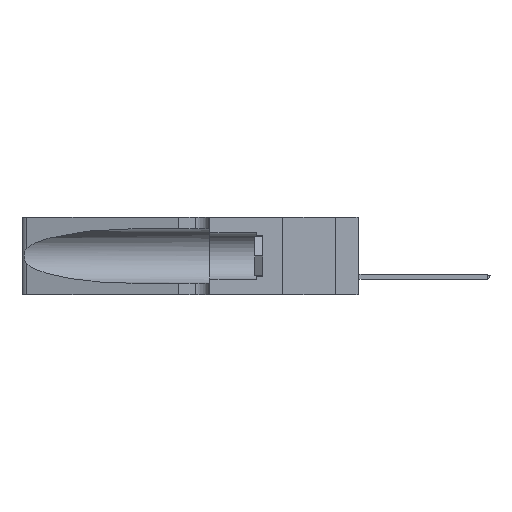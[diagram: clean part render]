
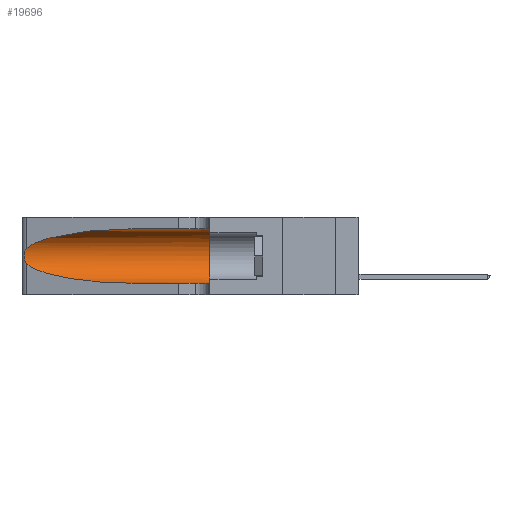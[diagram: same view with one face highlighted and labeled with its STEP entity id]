
A CAD part, left-side view. The second image highlights one B-rep face of the part: STEP entity #19696.
In plain terms, the highlighted cylindrical face has radius 3.308 mm (diameter 6.617 mm), a partial arc.
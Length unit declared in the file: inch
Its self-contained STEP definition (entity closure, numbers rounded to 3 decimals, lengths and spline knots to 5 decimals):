
#3224 = EDGE_CURVE ( 'NONE', #7602, #28068, #20324, .T. ) ;
#3632 = VERTEX_POINT ( 'NONE', #48541 ) ;
#4556 = EDGE_CURVE ( 'NONE', #50228, #3632, #8277, .T. ) ;
#5064 = DIRECTION ( 'NONE',  ( 0., 0., -1. ) ) ;
#5719 = FACE_OUTER_BOUND ( 'NONE', #31353, .T. ) ;
#6434 = CARTESIAN_POINT ( 'NONE',  ( 0.25639, 1.23184, 0.21858 ) ) ;
#6555 = AXIS2_PLACEMENT_3D ( 'NONE', #33342, #36722, #5064 ) ;
#7181 = DIRECTION ( 'NONE',  ( 0., -1., 0. ) ) ;
#7602 = VERTEX_POINT ( 'NONE', #30326 ) ;
#8277 = CIRCLE ( 'NONE', #33257, 0.13025 ) ;
#11417 = CARTESIAN_POINT ( 'NONE',  ( 0.18966, 0.96281, 0.05475 ) ) ;
#11422 = VECTOR ( 'NONE', #7181, 39.37008 ) ;
#12770 = VECTOR ( 'NONE', #43205, 39.37008 ) ;
#13550 = CARTESIAN_POINT ( 'NONE',  ( 0.2373, 1.15595, 0.28018 ) ) ;
#14125 = CARTESIAN_POINT ( 'NONE',  ( 0.25487, 1.22718, 0.22369 ) ) ;
#15288 = CARTESIAN_POINT ( 'NONE',  ( 0.1305, 1.61858, 0.31525 ) ) ;
#15460 = CARTESIAN_POINT ( 'NONE',  ( 0.25487, 1.22718, 0.14631 ) ) ;
#16062 = VERTEX_POINT ( 'NONE', #21186 ) ;
#16870 = CARTESIAN_POINT ( 'NONE',  ( 0.25639, 1.23186, 0.15144 ) ) ;
#19055 = CARTESIAN_POINT ( 'NONE',  ( 0.25854, 1.2359, 0.20912 ) ) ;
#19230 = CARTESIAN_POINT ( 'NONE',  ( 0.26075, 1.23896, 0.178 ) ) ;
#19696 = ADVANCED_FACE ( 'NONE', ( #5719 ), #38293, .F. ) ;
#19791 = ORIENTED_EDGE ( 'NONE', *, *, #4556, .F. ) ;
#20324 =( BOUNDED_CURVE ( )  B_SPLINE_CURVE ( 3, ( #29430, #41695, #13550, #21571 ),
 .UNSPECIFIED., .F., .F. ) 
 B_SPLINE_CURVE_WITH_KNOTS ( ( 4, 4 ),
 ( 1.5708, 2.84003 ),
 .UNSPECIFIED. ) 
 CURVE ( )  GEOMETRIC_REPRESENTATION_ITEM ( )  RATIONAL_B_SPLINE_CURVE ( ( 1., 0.87, 0.87, 1. ) ) 
 REPRESENTATION_ITEM ( '' )  );
#20940 =( BOUNDED_CURVE ( )  B_SPLINE_CURVE ( 3, ( #15460, #39589, #11417, #39419 ),
 .UNSPECIFIED., .F., .F. ) 
 B_SPLINE_CURVE_WITH_KNOTS ( ( 4, 4 ),
 ( 3.44316, 4.71239 ),
 .UNSPECIFIED. ) 
 CURVE ( )  GEOMETRIC_REPRESENTATION_ITEM ( )  RATIONAL_B_SPLINE_CURVE ( ( 1., 0.87, 0.87, 1. ) ) 
 REPRESENTATION_ITEM ( '' )  );
#21186 = CARTESIAN_POINT ( 'NONE',  ( 0.1305, 0.72297, 0.05475 ) ) ;
#21363 = EDGE_CURVE ( 'NONE', #28068, #22759, #41120, .T. ) ;
#21571 = CARTESIAN_POINT ( 'NONE',  ( 0.25487, 1.22718, 0.22369 ) ) ;
#22495 = ORIENTED_EDGE ( 'NONE', *, *, #44937, .T. ) ;
#22759 = VERTEX_POINT ( 'NONE', #25134 ) ;
#23254 = CARTESIAN_POINT ( 'NONE',  ( 0.25856, 1.23593, 0.16098 ) ) ;
#25134 = CARTESIAN_POINT ( 'NONE',  ( 0.25487, 1.22718, 0.14631 ) ) ;
#26694 = CARTESIAN_POINT ( 'NONE',  ( 0.26075, 1.23896, 0.19203 ) ) ;
#27233 = LINE ( 'NONE', #15288, #12770 ) ;
#28068 = VERTEX_POINT ( 'NONE', #39539 ) ;
#29221 = ORIENTED_EDGE ( 'NONE', *, *, #3224, .T. ) ;
#29430 = CARTESIAN_POINT ( 'NONE',  ( 0.1305, 0.72297, 0.31525 ) ) ;
#30326 = CARTESIAN_POINT ( 'NONE',  ( 0.1305, 0.72297, 0.31525 ) ) ;
#31324 = CARTESIAN_POINT ( 'NONE',  ( 0.1305, 0.35, 0.185 ) ) ;
#31353 = EDGE_LOOP ( 'NONE', ( #29221, #44229, #22495, #33733, #19791, #46419 ) ) ;
#31357 = CARTESIAN_POINT ( 'NONE',  ( 0.1305, 1.61858, 0.05475 ) ) ;
#33257 = AXIS2_PLACEMENT_3D ( 'NONE', #31324, #39546, #50849 ) ;
#33342 = CARTESIAN_POINT ( 'NONE',  ( 0.1305, 1.61858, 0.185 ) ) ;
#33733 = ORIENTED_EDGE ( 'NONE', *, *, #48502, .T. ) ;
#34178 = CARTESIAN_POINT ( 'NONE',  ( 0.25555, 1.22993, 0.14849 ) ) ;
#36722 = DIRECTION ( 'NONE',  ( 0., -1., 0. ) ) ;
#37525 = CARTESIAN_POINT ( 'NONE',  ( 0.25787, 1.23484, 0.2124 ) ) ;
#38264 = CARTESIAN_POINT ( 'NONE',  ( 0.25555, 1.22994, 0.2215 ) ) ;
#38293 = CYLINDRICAL_SURFACE ( 'NONE', #6555, 0.13025 ) ;
#38805 = CARTESIAN_POINT ( 'NONE',  ( 0.26018, 1.23835, 0.19895 ) ) ;
#39419 = CARTESIAN_POINT ( 'NONE',  ( 0.1305, 0.72297, 0.05475 ) ) ;
#39489 = CARTESIAN_POINT ( 'NONE',  ( 0.25487, 1.22718, 0.14631 ) ) ;
#39539 = CARTESIAN_POINT ( 'NONE',  ( 0.25487, 1.22718, 0.22369 ) ) ;
#39546 = DIRECTION ( 'NONE',  ( 0., 1., 0. ) ) ;
#39589 = CARTESIAN_POINT ( 'NONE',  ( 0.2373, 1.15595, 0.08982 ) ) ;
#41120 = B_SPLINE_CURVE_WITH_KNOTS ( 'NONE', 3,
 ( #14125, #38264, #6434, #37525, #19055, #38805, #26694, #19230, #47148, #23254, #51180, #16870, #34178, #39489 ),
 .UNSPECIFIED., .F., .F.,
 ( 4, 2, 2, 2, 2, 2, 4 ),
 ( 0., 0.00027, 0.00053, 0.00107, 0.0016, 0.00187, 0.00214 ),
 .UNSPECIFIED. ) ;
#41695 = CARTESIAN_POINT ( 'NONE',  ( 0.18966, 0.96281, 0.31525 ) ) ;
#43205 = DIRECTION ( 'NONE',  ( 0., -1., 0. ) ) ;
#44229 = ORIENTED_EDGE ( 'NONE', *, *, #21363, .T. ) ;
#44937 = EDGE_CURVE ( 'NONE', #22759, #16062, #20940, .T. ) ;
#45005 = EDGE_CURVE ( 'NONE', #7602, #50228, #27233, .T. ) ;
#46419 = ORIENTED_EDGE ( 'NONE', *, *, #45005, .F. ) ;
#47148 = CARTESIAN_POINT ( 'NONE',  ( 0.26017, 1.23833, 0.17102 ) ) ;
#48502 = EDGE_CURVE ( 'NONE', #16062, #3632, #48819, .T. ) ;
#48541 = CARTESIAN_POINT ( 'NONE',  ( 0.1305, 0.35, 0.05475 ) ) ;
#48819 = LINE ( 'NONE', #31357, #11422 ) ;
#50228 = VERTEX_POINT ( 'NONE', #51059 ) ;
#50849 = DIRECTION ( 'NONE',  ( 0., 0., 1. ) ) ;
#51059 = CARTESIAN_POINT ( 'NONE',  ( 0.1305, 0.35, 0.31525 ) ) ;
#51180 = CARTESIAN_POINT ( 'NONE',  ( 0.25789, 1.23486, 0.15765 ) ) ;
